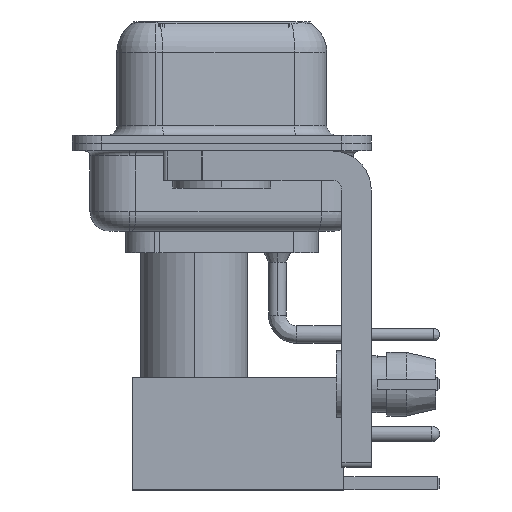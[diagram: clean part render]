
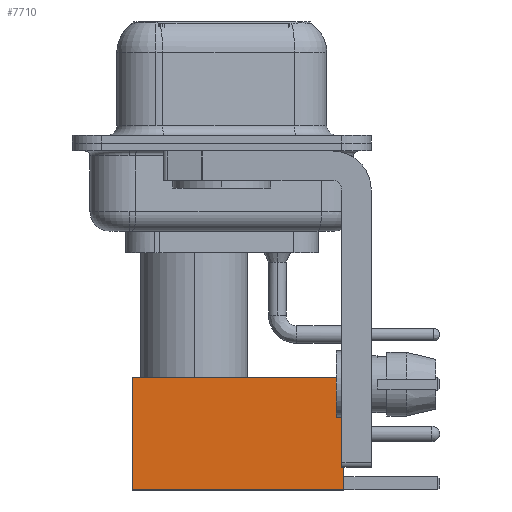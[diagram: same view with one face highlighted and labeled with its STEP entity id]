
A CAD part, left-side view. The second image highlights one B-rep face of the part: STEP entity #7710.
In plain terms, the highlighted face is planar.
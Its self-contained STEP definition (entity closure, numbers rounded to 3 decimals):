
#28 = DIRECTION ( 'NONE',  ( 0., 0., -1. ) ) ;
#2934 = PLANE ( 'NONE',  #9488 ) ;
#4957 = CARTESIAN_POINT ( 'NONE',  ( 2.875, 2.875, 0. ) ) ;
#5474 = VECTOR ( 'NONE', #28, 1000. ) ;
#6008 = CARTESIAN_POINT ( 'NONE',  ( -2.875, 2.875, 0. ) ) ;
#6807 = FACE_OUTER_BOUND ( 'NONE', #8981, .T. ) ;
#6859 = VERTEX_POINT ( 'NONE', #19790 ) ;
#7710 = ADVANCED_FACE ( 'NONE', ( #6807 ), #2934, .T. ) ;
#8981 = EDGE_LOOP ( 'NONE', ( #22812, #9794, #10571, #27186 ) ) ;
#9488 = AXIS2_PLACEMENT_3D ( 'NONE', #16007, #22479, #24470 ) ;
#9794 = ORIENTED_EDGE ( 'NONE', *, *, #14899, .T. ) ;
#9890 = EDGE_CURVE ( 'NONE', #6859, #20818, #11963, .T. ) ;
#10388 = DIRECTION ( 'NONE',  ( -1., 0., 0. ) ) ;
#10571 = ORIENTED_EDGE ( 'NONE', *, *, #11132, .F. ) ;
#11052 = CARTESIAN_POINT ( 'NONE',  ( 2.875, 2.875, 0. ) ) ;
#11132 = EDGE_CURVE ( 'NONE', #20818, #12390, #15052, .T. ) ;
#11963 = LINE ( 'NONE', #18732, #25104 ) ;
#12390 = VERTEX_POINT ( 'NONE', #26196 ) ;
#12902 = LINE ( 'NONE', #11052, #5474 ) ;
#14545 = CARTESIAN_POINT ( 'NONE',  ( 0., 2.875, 0. ) ) ;
#14755 = DIRECTION ( 'NONE',  ( 0., 0., -1. ) ) ;
#14899 = EDGE_CURVE ( 'NONE', #25064, #12390, #25778, .T. ) ;
#15052 = LINE ( 'NONE', #6008, #25190 ) ;
#16007 = CARTESIAN_POINT ( 'NONE',  ( 2.875, 2.875, 0. ) ) ;
#17007 = VECTOR ( 'NONE', #10388, 1000. ) ;
#17997 = CARTESIAN_POINT ( 'NONE',  ( -2.875, 2.875, 10.82 ) ) ;
#18567 = EDGE_CURVE ( 'NONE', #6859, #25064, #12902, .T. ) ;
#18732 = CARTESIAN_POINT ( 'NONE',  ( 0., 2.875, 10.82 ) ) ;
#19790 = CARTESIAN_POINT ( 'NONE',  ( 2.875, 2.875, 10.82 ) ) ;
#20745 = DIRECTION ( 'NONE',  ( -1., 0., 0. ) ) ;
#20818 = VERTEX_POINT ( 'NONE', #17997 ) ;
#22479 = DIRECTION ( 'NONE',  ( 0., 1., 0. ) ) ;
#22812 = ORIENTED_EDGE ( 'NONE', *, *, #18567, .T. ) ;
#24470 = DIRECTION ( 'NONE',  ( 0., 0., 1. ) ) ;
#25064 = VERTEX_POINT ( 'NONE', #4957 ) ;
#25104 = VECTOR ( 'NONE', #20745, 1000. ) ;
#25190 = VECTOR ( 'NONE', #14755, 1000. ) ;
#25778 = LINE ( 'NONE', #14545, #17007 ) ;
#26196 = CARTESIAN_POINT ( 'NONE',  ( -2.875, 2.875, 0. ) ) ;
#27186 = ORIENTED_EDGE ( 'NONE', *, *, #9890, .F. ) ;
